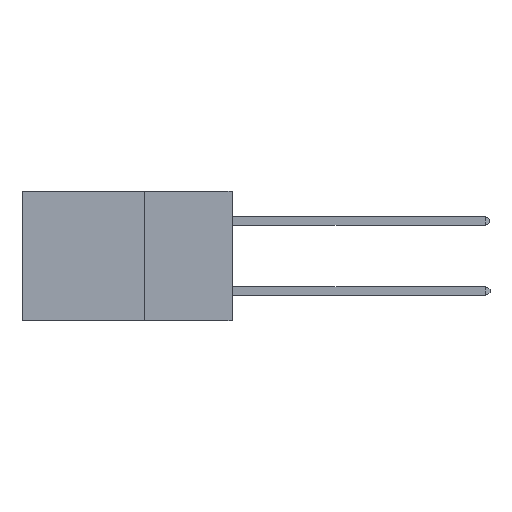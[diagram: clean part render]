
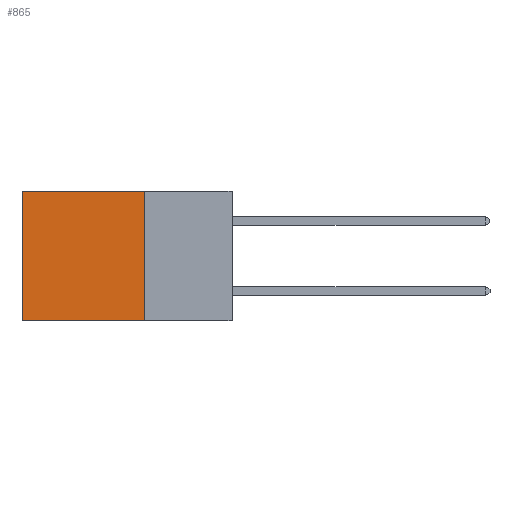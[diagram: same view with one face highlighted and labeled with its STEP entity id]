
A CAD part, left-side view. The second image highlights one B-rep face of the part: STEP entity #865.
In plain terms, the highlighted planar face has unit normal (-1, 0, 0).
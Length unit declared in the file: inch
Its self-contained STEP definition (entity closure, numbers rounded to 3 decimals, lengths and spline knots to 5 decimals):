
#74 = CARTESIAN_POINT ( 'NONE',  ( 0.2875, 0.25, 0. ) ) ;
#133 = CARTESIAN_POINT ( 'NONE',  ( 0.2875, 0.25, 0. ) ) ;
#149 = AXIS2_PLACEMENT_3D ( 'NONE', #74, #10514, #1626 ) ;
#202 = CARTESIAN_POINT ( 'NONE',  ( 0.2875, 0.6, -0.37 ) ) ;
#865 = ADVANCED_FACE ( 'NONE', ( #8339 ), #13383, .F. ) ;
#1254 = EDGE_CURVE ( 'NONE', #10068, #5420, #9232, .T. ) ;
#1626 = DIRECTION ( 'NONE',  ( 0., 0., -1. ) ) ;
#2628 = EDGE_LOOP ( 'NONE', ( #13248, #6487, #7260, #8296 ) ) ;
#3783 = LINE ( 'NONE', #133, #18750 ) ;
#4743 = CARTESIAN_POINT ( 'NONE',  ( 0.2875, 0.25, 0. ) ) ;
#4762 = DIRECTION ( 'NONE',  ( 0., 0., -1. ) ) ;
#5326 = VECTOR ( 'NONE', #11337, 39.37008 ) ;
#5420 = VERTEX_POINT ( 'NONE', #202 ) ;
#6487 = ORIENTED_EDGE ( 'NONE', *, *, #1254, .F. ) ;
#7166 = CARTESIAN_POINT ( 'NONE',  ( 0.2875, 0.6, 0. ) ) ;
#7260 = ORIENTED_EDGE ( 'NONE', *, *, #7574, .F. ) ;
#7491 = LINE ( 'NONE', #16852, #10861 ) ;
#7574 = EDGE_CURVE ( 'NONE', #10266, #10068, #3783, .T. ) ;
#8254 = EDGE_CURVE ( 'NONE', #10266, #10107, #8368, .T. ) ;
#8296 = ORIENTED_EDGE ( 'NONE', *, *, #8254, .T. ) ;
#8339 = FACE_OUTER_BOUND ( 'NONE', #2628, .T. ) ;
#8368 = LINE ( 'NONE', #4743, #18948 ) ;
#9232 = LINE ( 'NONE', #18499, #5326 ) ;
#9694 = DIRECTION ( 'NONE',  ( 0., 0., -1. ) ) ;
#10068 = VERTEX_POINT ( 'NONE', #12807 ) ;
#10107 = VERTEX_POINT ( 'NONE', #7166 ) ;
#10266 = VERTEX_POINT ( 'NONE', #13301 ) ;
#10514 = DIRECTION ( 'NONE',  ( 1., 0., 0. ) ) ;
#10861 = VECTOR ( 'NONE', #9694, 39.37008 ) ;
#11337 = DIRECTION ( 'NONE',  ( 0., 1., 0. ) ) ;
#12807 = CARTESIAN_POINT ( 'NONE',  ( 0.2875, 0.25, -0.37 ) ) ;
#13248 = ORIENTED_EDGE ( 'NONE', *, *, #16754, .T. ) ;
#13301 = CARTESIAN_POINT ( 'NONE',  ( 0.2875, 0.25, 0. ) ) ;
#13383 = PLANE ( 'NONE',  #149 ) ;
#14933 = DIRECTION ( 'NONE',  ( 0., 1., 0. ) ) ;
#16754 = EDGE_CURVE ( 'NONE', #10107, #5420, #7491, .T. ) ;
#16852 = CARTESIAN_POINT ( 'NONE',  ( 0.2875, 0.6, 0. ) ) ;
#18499 = CARTESIAN_POINT ( 'NONE',  ( 0.2875, 0.25, -0.37 ) ) ;
#18750 = VECTOR ( 'NONE', #4762, 39.37008 ) ;
#18948 = VECTOR ( 'NONE', #14933, 39.37008 ) ;
